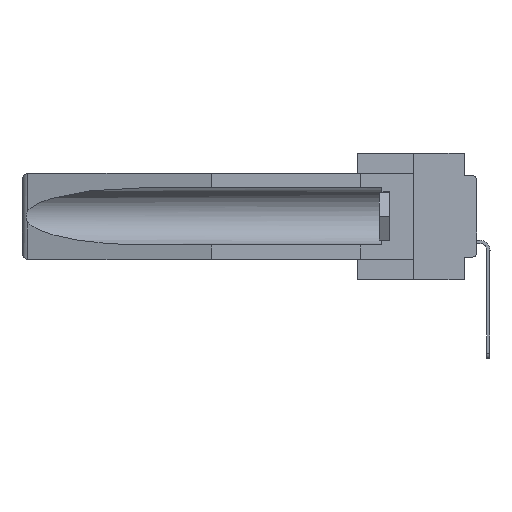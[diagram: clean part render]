
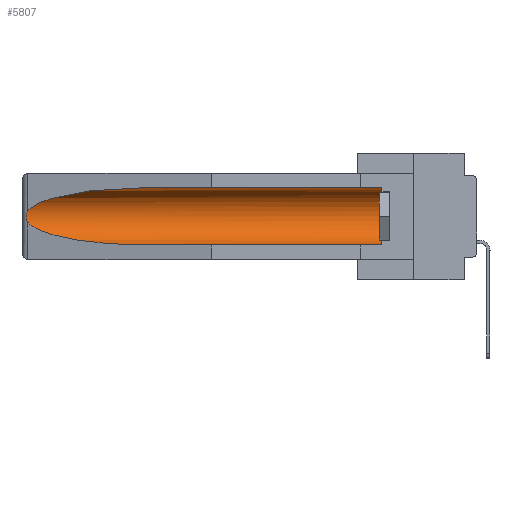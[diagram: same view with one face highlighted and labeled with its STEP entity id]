
A CAD part, left-side view. The second image highlights one B-rep face of the part: STEP entity #5807.
In plain terms, the highlighted cylindrical face has radius 2.857 mm (diameter 5.715 mm), a partial arc.
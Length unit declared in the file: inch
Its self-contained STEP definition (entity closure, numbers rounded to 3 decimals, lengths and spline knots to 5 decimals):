
#620 = ORIENTED_EDGE ( 'NONE', *, *, #28333, .T. ) ;
#1085 = CARTESIAN_POINT ( 'NONE',  ( 0.2675, 1.53308, -0.16763 ) ) ;
#2689 = DIRECTION ( 'NONE',  ( 0., 0., 1. ) ) ;
#3832 = VERTEX_POINT ( 'NONE', #27194 ) ;
#4017 = CARTESIAN_POINT ( 'NONE',  ( 0.25451, 1.48313, -0.24835 ) ) ;
#4625 = B_SPLINE_CURVE_WITH_KNOTS ( 'NONE', 3,
 ( #23610, #23437, #17664, #6523, #1085, #20387, #28674, #20556, #7042, #9202 ),
 .UNSPECIFIED., .F., .F.,
 ( 4, 2, 2, 2, 4 ),
 ( 0., 0.00029, 0.00058, 0.00087, 0.00117 ),
 .UNSPECIFIED. ) ;
#4916 = VERTEX_POINT ( 'NONE', #29156 ) ;
#5266 = AXIS2_PLACEMENT_3D ( 'NONE', #17514, #13847, #2689 ) ;
#5437 = LINE ( 'NONE', #11485, #14055 ) ;
#5737 = VERTEX_POINT ( 'NONE', #17529 ) ;
#5807 = ADVANCED_FACE ( 'NONE', ( #30096 ), #25208, .F. ) ;
#6523 = CARTESIAN_POINT ( 'NONE',  ( 0.2673, 1.5327, -0.16383 ) ) ;
#7042 = CARTESIAN_POINT ( 'NONE',  ( 0.26597, 1.5296, -0.19026 ) ) ;
#8587 = CARTESIAN_POINT ( 'NONE',  ( 0.155, 1.07973, -0.059 ) ) ;
#9202 = CARTESIAN_POINT ( 'NONE',  ( 0.26537, 1.52718, -0.19328 ) ) ;
#10982 = ORIENTED_EDGE ( 'NONE', *, *, #11253, .F. ) ;
#11253 = EDGE_CURVE ( 'NONE', #3832, #20915, #17552, .T. ) ;
#11485 = CARTESIAN_POINT ( 'NONE',  ( 0.155, -0.30754, -0.059 ) ) ;
#11861 = EDGE_CURVE ( 'NONE', #20651, #5737, #34588, .T. ) ;
#11926 = CARTESIAN_POINT ( 'NONE',  ( 0.155, 0.126, -0.1715 ) ) ;
#12151 = DIRECTION ( 'NONE',  ( 0., 1., 0. ) ) ;
#12529 = ORIENTED_EDGE ( 'NONE', *, *, #30633, .T. ) ;
#13114 = CARTESIAN_POINT ( 'NONE',  ( 0.155, 1.07973, -0.059 ) ) ;
#13833 = CARTESIAN_POINT ( 'NONE',  ( 0.25451, 1.48313, -0.09465 ) ) ;
#13847 = DIRECTION ( 'NONE',  ( 0., 1., 0. ) ) ;
#14055 = VECTOR ( 'NONE', #21813, 39.37008 ) ;
#14820 = CARTESIAN_POINT ( 'NONE',  ( 0.155, 1.07973, -0.284 ) ) ;
#16354 = AXIS2_PLACEMENT_3D ( 'NONE', #11926, #17861, #31255 ) ;
#17094 = VECTOR ( 'NONE', #12151, 39.37008 ) ;
#17514 = CARTESIAN_POINT ( 'NONE',  ( 0.155, -0.30754, -0.1715 ) ) ;
#17529 = CARTESIAN_POINT ( 'NONE',  ( 0.26537, 1.52718, -0.14972 ) ) ;
#17552 = LINE ( 'NONE', #28917, #17094 ) ;
#17664 = CARTESIAN_POINT ( 'NONE',  ( 0.26654, 1.53092, -0.15636 ) ) ;
#17861 = DIRECTION ( 'NONE',  ( 0., -1., 0. ) ) ;
#18278 = CARTESIAN_POINT ( 'NONE',  ( 0.155, 1.07973, -0.284 ) ) ;
#18707 = CARTESIAN_POINT ( 'NONE',  ( 0.26537, 1.52718, -0.14972 ) ) ;
#20135 = CARTESIAN_POINT ( 'NONE',  ( 0.26537, 1.52718, -0.19328 ) ) ;
#20387 = CARTESIAN_POINT ( 'NONE',  ( 0.2675, 1.53308, -0.17534 ) ) ;
#20556 = CARTESIAN_POINT ( 'NONE',  ( 0.26655, 1.53094, -0.18657 ) ) ;
#20589 = CARTESIAN_POINT ( 'NONE',  ( 0.26537, 1.52718, -0.19328 ) ) ;
#20651 = VERTEX_POINT ( 'NONE', #8587 ) ;
#20915 = VERTEX_POINT ( 'NONE', #18278 ) ;
#21425 = CARTESIAN_POINT ( 'NONE',  ( 0.21114, 1.30732, -0.059 ) ) ;
#21813 = DIRECTION ( 'NONE',  ( 0., 1., 0. ) ) ;
#23320 = ORIENTED_EDGE ( 'NONE', *, *, #33237, .T. ) ;
#23364 = VERTEX_POINT ( 'NONE', #20135 ) ;
#23437 = CARTESIAN_POINT ( 'NONE',  ( 0.26597, 1.52961, -0.15275 ) ) ;
#23610 = CARTESIAN_POINT ( 'NONE',  ( 0.26537, 1.52718, -0.14972 ) ) ;
#23796 = EDGE_LOOP ( 'NONE', ( #31233, #23320, #12529, #10982, #30245, #620 ) ) ;
#25208 = CYLINDRICAL_SURFACE ( 'NONE', #5266, 0.1125 ) ;
#26730 = CIRCLE ( 'NONE', #16354, 0.1125 ) ;
#26982 =( BOUNDED_CURVE ( )  B_SPLINE_CURVE ( 3, ( #20589, #4017, #31612, #14820 ),
 .UNSPECIFIED., .F., .F. ) 
 B_SPLINE_CURVE_WITH_KNOTS ( ( 4, 4 ),
 ( 0.1948, 1.5708 ),
 .UNSPECIFIED. ) 
 CURVE ( )  GEOMETRIC_REPRESENTATION_ITEM ( )  RATIONAL_B_SPLINE_CURVE ( ( 1., 0.848, 0.848, 1. ) ) 
 REPRESENTATION_ITEM ( '' )  );
#27194 = CARTESIAN_POINT ( 'NONE',  ( 0.155, 0.126, -0.284 ) ) ;
#28128 = EDGE_CURVE ( 'NONE', #3832, #4916, #26730, .T. ) ;
#28333 = EDGE_CURVE ( 'NONE', #4916, #20651, #5437, .T. ) ;
#28674 = CARTESIAN_POINT ( 'NONE',  ( 0.2673, 1.53269, -0.17917 ) ) ;
#28917 = CARTESIAN_POINT ( 'NONE',  ( 0.155, -0.30754, -0.284 ) ) ;
#29156 = CARTESIAN_POINT ( 'NONE',  ( 0.155, 0.126, -0.059 ) ) ;
#30096 = FACE_OUTER_BOUND ( 'NONE', #23796, .T. ) ;
#30245 = ORIENTED_EDGE ( 'NONE', *, *, #28128, .T. ) ;
#30633 = EDGE_CURVE ( 'NONE', #23364, #20915, #26982, .T. ) ;
#31233 = ORIENTED_EDGE ( 'NONE', *, *, #11861, .T. ) ;
#31255 = DIRECTION ( 'NONE',  ( 0., 0., 1. ) ) ;
#31612 = CARTESIAN_POINT ( 'NONE',  ( 0.21114, 1.30732, -0.284 ) ) ;
#33237 = EDGE_CURVE ( 'NONE', #5737, #23364, #4625, .T. ) ;
#34588 =( BOUNDED_CURVE ( )  B_SPLINE_CURVE ( 3, ( #13114, #21425, #13833, #18707 ),
 .UNSPECIFIED., .F., .F. ) 
 B_SPLINE_CURVE_WITH_KNOTS ( ( 4, 4 ),
 ( 4.71239, 6.08839 ),
 .UNSPECIFIED. ) 
 CURVE ( )  GEOMETRIC_REPRESENTATION_ITEM ( )  RATIONAL_B_SPLINE_CURVE ( ( 1., 0.848, 0.848, 1. ) ) 
 REPRESENTATION_ITEM ( '' )  );
